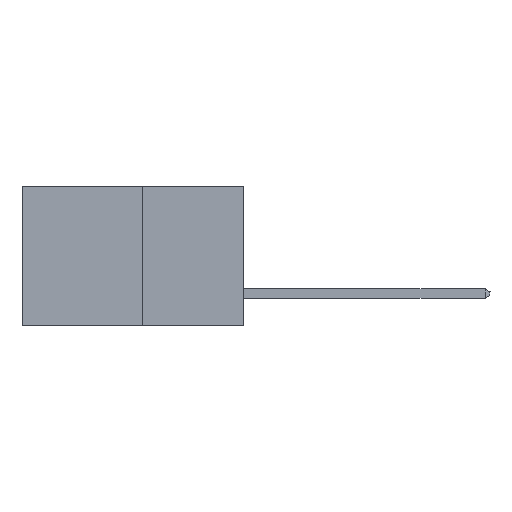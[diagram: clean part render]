
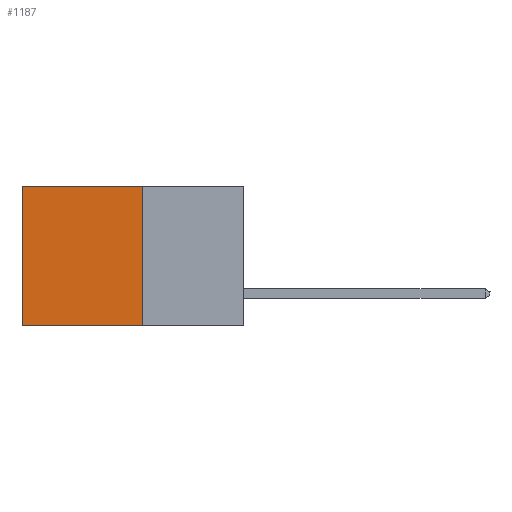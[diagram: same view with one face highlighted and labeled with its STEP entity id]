
A CAD part, left-side view. The second image highlights one B-rep face of the part: STEP entity #1187.
In plain terms, the highlighted planar face has unit normal (-1, 0, 0).
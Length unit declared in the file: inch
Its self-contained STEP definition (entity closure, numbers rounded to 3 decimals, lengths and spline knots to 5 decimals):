
#110 = ORIENTED_EDGE ( 'NONE', *, *, #2448, .F. ) ;
#280 = VECTOR ( 'NONE', #1452, 39.37008 ) ;
#1187 = ADVANCED_FACE ( 'NONE', ( #6377 ), #3474, .F. ) ;
#1438 = CARTESIAN_POINT ( 'NONE',  ( 0.277, 0.27, -0.37 ) ) ;
#1452 = DIRECTION ( 'NONE',  ( 0., 1., 0. ) ) ;
#1795 = EDGE_CURVE ( 'NONE', #11892, #11744, #4364, .T. ) ;
#2448 = EDGE_CURVE ( 'NONE', #11892, #3654, #9546, .T. ) ;
#3330 = EDGE_CURVE ( 'NONE', #11744, #8756, #13072, .T. ) ;
#3474 = PLANE ( 'NONE',  #15932 ) ;
#3654 = VERTEX_POINT ( 'NONE', #1438 ) ;
#3764 = EDGE_LOOP ( 'NONE', ( #18565, #11332, #110, #4211 ) ) ;
#4211 = ORIENTED_EDGE ( 'NONE', *, *, #1795, .T. ) ;
#4364 = LINE ( 'NONE', #9629, #280 ) ;
#6377 = FACE_OUTER_BOUND ( 'NONE', #3764, .T. ) ;
#6597 = CARTESIAN_POINT ( 'NONE',  ( 0.277, 0.27, 0. ) ) ;
#6716 = LINE ( 'NONE', #18664, #7205 ) ;
#7205 = VECTOR ( 'NONE', #9938, 39.37008 ) ;
#8350 = DIRECTION ( 'NONE',  ( 0., 0., -1. ) ) ;
#8756 = VERTEX_POINT ( 'NONE', #11165 ) ;
#9546 = LINE ( 'NONE', #11397, #13105 ) ;
#9629 = CARTESIAN_POINT ( 'NONE',  ( 0.277, 0.27, 0. ) ) ;
#9938 = DIRECTION ( 'NONE',  ( 0., 1., 0. ) ) ;
#10030 = CARTESIAN_POINT ( 'NONE',  ( 0.277, 0.59, -0.37 ) ) ;
#11165 = CARTESIAN_POINT ( 'NONE',  ( 0.277, 0.59, -0.37 ) ) ;
#11332 = ORIENTED_EDGE ( 'NONE', *, *, #11373, .F. ) ;
#11373 = EDGE_CURVE ( 'NONE', #3654, #8756, #6716, .T. ) ;
#11397 = CARTESIAN_POINT ( 'NONE',  ( 0.277, 0.27, -0.37 ) ) ;
#11536 = DIRECTION ( 'NONE',  ( 0., 0., -1. ) ) ;
#11744 = VERTEX_POINT ( 'NONE', #12278 ) ;
#11892 = VERTEX_POINT ( 'NONE', #6597 ) ;
#12278 = CARTESIAN_POINT ( 'NONE',  ( 0.277, 0.59, 0. ) ) ;
#12629 = VECTOR ( 'NONE', #8350, 39.37008 ) ;
#13072 = LINE ( 'NONE', #10030, #12629 ) ;
#13105 = VECTOR ( 'NONE', #11536, 39.37008 ) ;
#14194 = DIRECTION ( 'NONE',  ( 0., 0., -1. ) ) ;
#14904 = CARTESIAN_POINT ( 'NONE',  ( 0.277, 0.27, -0.37 ) ) ;
#15112 = DIRECTION ( 'NONE',  ( 1., 0., 0. ) ) ;
#15932 = AXIS2_PLACEMENT_3D ( 'NONE', #14904, #15112, #14194 ) ;
#18565 = ORIENTED_EDGE ( 'NONE', *, *, #3330, .T. ) ;
#18664 = CARTESIAN_POINT ( 'NONE',  ( 0.277, 0.27, -0.37 ) ) ;
